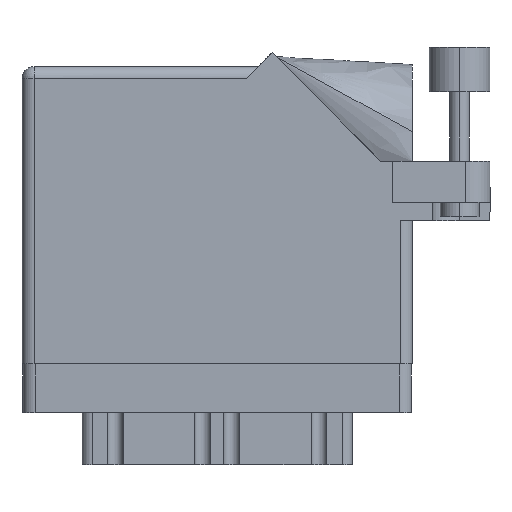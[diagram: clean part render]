
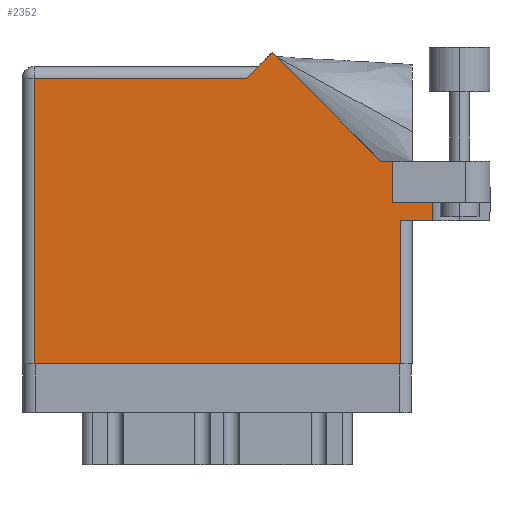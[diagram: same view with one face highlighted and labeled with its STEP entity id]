
A CAD part, front view. The second image highlights one B-rep face of the part: STEP entity #2352.
In plain terms, the highlighted face is planar.
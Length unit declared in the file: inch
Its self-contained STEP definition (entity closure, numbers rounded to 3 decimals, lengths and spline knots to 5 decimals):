
#315 = VERTEX_POINT ( 'NONE', #24231 ) ;
#578 = CARTESIAN_POINT ( 'NONE',  ( 1.155, 1.468, 0. ) ) ;
#921 = VERTEX_POINT ( 'NONE', #22400 ) ;
#976 = LINE ( 'NONE', #22211, #2198 ) ;
#1075 = CARTESIAN_POINT ( 'NONE',  ( 0.062, 0., 0. ) ) ;
#1170 = AXIS2_PLACEMENT_3D ( 'NONE', #5029, #34417, #10353 ) ;
#1180 = VERTEX_POINT ( 'NONE', #21303 ) ;
#1255 = LINE ( 'NONE', #20189, #10059 ) ;
#1613 = EDGE_CURVE ( 'NONE', #1180, #15793, #21962, .T. ) ;
#2024 = LINE ( 'NONE', #17772, #23167 ) ;
#2198 = VECTOR ( 'NONE', #30543, 39.37008 ) ;
#2352 = ADVANCED_FACE ( 'NONE', ( #12845 ), #23617, .F. ) ;
#2527 = DIRECTION ( 'NONE',  ( 0., 1., 0. ) ) ;
#2642 = VECTOR ( 'NONE', #23345, 39.37008 ) ;
#2678 = CARTESIAN_POINT ( 'NONE',  ( 0., 0., 0. ) ) ;
#2795 = CARTESIAN_POINT ( 'NONE',  ( 1.84442, 1.044, 0. ) ) ;
#3023 = CARTESIAN_POINT ( 'NONE',  ( 0.062, 0., 0. ) ) ;
#3387 = EDGE_CURVE ( 'NONE', #32485, #20541, #27053, .T. ) ;
#4125 = LINE ( 'NONE', #12821, #17783 ) ;
#4178 = ORIENTED_EDGE ( 'NONE', *, *, #29573, .T. ) ;
#4871 = ORIENTED_EDGE ( 'NONE', *, *, #3387, .T. ) ;
#5029 = CARTESIAN_POINT ( 'NONE',  ( 0., 1.53, 0. ) ) ;
#5056 = EDGE_CURVE ( 'NONE', #9277, #1180, #976, .T. ) ;
#5704 = CARTESIAN_POINT ( 'NONE',  ( 1.217, 1.53, 0. ) ) ;
#5858 = DIRECTION ( 'NONE',  ( 1., 0., 0. ) ) ;
#6406 = EDGE_CURVE ( 'NONE', #921, #31021, #2024, .T. ) ;
#6915 = CARTESIAN_POINT ( 'NONE',  ( 1.91, 1.044, 0. ) ) ;
#7485 = LINE ( 'NONE', #9984, #20036 ) ;
#8009 = DIRECTION ( 'NONE',  ( -0.707, -0.707, 0. ) ) ;
#8071 = VERTEX_POINT ( 'NONE', #6915 ) ;
#8391 = ORIENTED_EDGE ( 'NONE', *, *, #23736, .F. ) ;
#8511 = VECTOR ( 'NONE', #13611, 39.37008 ) ;
#8590 = DIRECTION ( 'NONE',  ( -1., 0., 0. ) ) ;
#8697 = DIRECTION ( 'NONE',  ( 0., 1., 0. ) ) ;
#9277 = VERTEX_POINT ( 'NONE', #578 ) ;
#9984 = CARTESIAN_POINT ( 'NONE',  ( 1.948, 0.737, 0. ) ) ;
#10059 = VECTOR ( 'NONE', #8697, 39.37008 ) ;
#10234 = CARTESIAN_POINT ( 'NONE',  ( 1.84442, 1.044, 0. ) ) ;
#10353 = DIRECTION ( 'NONE',  ( -1., 0., 0. ) ) ;
#12574 = CARTESIAN_POINT ( 'NONE',  ( 2.01, 0.737, 0. ) ) ;
#12821 = CARTESIAN_POINT ( 'NONE',  ( 2.1115, 1.16177, 0. ) ) ;
#12845 = FACE_OUTER_BOUND ( 'NONE', #19191, .T. ) ;
#13579 = ORIENTED_EDGE ( 'NONE', *, *, #19293, .T. ) ;
#13611 = DIRECTION ( 'NONE',  ( -0.707, 0.707, 0. ) ) ;
#14449 = VECTOR ( 'NONE', #8009, 39.37008 ) ;
#15306 = DIRECTION ( 'NONE',  ( 1., 0., 0. ) ) ;
#15793 = VERTEX_POINT ( 'NONE', #1075 ) ;
#16318 = DIRECTION ( 'NONE',  ( 0., -1., 0. ) ) ;
#16716 = CARTESIAN_POINT ( 'NONE',  ( 1.28771, 1.60071, 0. ) ) ;
#17705 = VECTOR ( 'NONE', #16318, 39.37008 ) ;
#17772 = CARTESIAN_POINT ( 'NONE',  ( 1.91, 0.831, 0. ) ) ;
#17783 = VECTOR ( 'NONE', #22886, 39.37008 ) ;
#18786 = LINE ( 'NONE', #2678, #30575 ) ;
#18927 = VECTOR ( 'NONE', #8590, 39.37008 ) ;
#19001 = LINE ( 'NONE', #5704, #14449 ) ;
#19191 = EDGE_LOOP ( 'NONE', ( #13579, #20153, #23503, #8391, #21828, #19923, #21890, #4871, #4178, #25066, #27024 ) ) ;
#19293 = EDGE_CURVE ( 'NONE', #15793, #315, #18786, .T. ) ;
#19923 = ORIENTED_EDGE ( 'NONE', *, *, #28394, .T. ) ;
#20036 = VECTOR ( 'NONE', #2527, 39.37008 ) ;
#20153 = ORIENTED_EDGE ( 'NONE', *, *, #34497, .T. ) ;
#20189 = CARTESIAN_POINT ( 'NONE',  ( 1.91, 0.831, 0. ) ) ;
#20541 = VERTEX_POINT ( 'NONE', #16716 ) ;
#20775 = VERTEX_POINT ( 'NONE', #30864 ) ;
#21303 = CARTESIAN_POINT ( 'NONE',  ( 0.062, 1.468, 0. ) ) ;
#21828 = ORIENTED_EDGE ( 'NONE', *, *, #6406, .F. ) ;
#21890 = ORIENTED_EDGE ( 'NONE', *, *, #23672, .T. ) ;
#21962 = LINE ( 'NONE', #3023, #17705 ) ;
#22211 = CARTESIAN_POINT ( 'NONE',  ( 0., 1.468, 0. ) ) ;
#22400 = CARTESIAN_POINT ( 'NONE',  ( 1.91, 0.831, 0. ) ) ;
#22886 = DIRECTION ( 'NONE',  ( 0., -1., 0. ) ) ;
#23167 = VECTOR ( 'NONE', #15306, 39.37008 ) ;
#23345 = DIRECTION ( 'NONE',  ( 1., 0., 0. ) ) ;
#23503 = ORIENTED_EDGE ( 'NONE', *, *, #27329, .T. ) ;
#23617 = PLANE ( 'NONE',  #1170 ) ;
#23672 = EDGE_CURVE ( 'NONE', #8071, #32485, #25218, .T. ) ;
#23736 = EDGE_CURVE ( 'NONE', #31021, #20775, #4125, .T. ) ;
#24231 = CARTESIAN_POINT ( 'NONE',  ( 1.948, 0., 0. ) ) ;
#25066 = ORIENTED_EDGE ( 'NONE', *, *, #5056, .T. ) ;
#25218 = LINE ( 'NONE', #32835, #18927 ) ;
#25669 = CARTESIAN_POINT ( 'NONE',  ( 1.948, 0.737, 0. ) ) ;
#26385 = LINE ( 'NONE', #12574, #2642 ) ;
#26763 = CARTESIAN_POINT ( 'NONE',  ( 2.1115, 0.831, 0. ) ) ;
#27024 = ORIENTED_EDGE ( 'NONE', *, *, #1613, .T. ) ;
#27053 = LINE ( 'NONE', #2795, #8511 ) ;
#27329 = EDGE_CURVE ( 'NONE', #31953, #20775, #26385, .T. ) ;
#28394 = EDGE_CURVE ( 'NONE', #921, #8071, #1255, .T. ) ;
#29573 = EDGE_CURVE ( 'NONE', #20541, #9277, #19001, .T. ) ;
#30543 = DIRECTION ( 'NONE',  ( -1., 0., 0. ) ) ;
#30575 = VECTOR ( 'NONE', #5858, 39.37008 ) ;
#30864 = CARTESIAN_POINT ( 'NONE',  ( 2.1115, 0.737, 0. ) ) ;
#31021 = VERTEX_POINT ( 'NONE', #26763 ) ;
#31953 = VERTEX_POINT ( 'NONE', #25669 ) ;
#32485 = VERTEX_POINT ( 'NONE', #10234 ) ;
#32835 = CARTESIAN_POINT ( 'NONE',  ( 2.41, 1.044, 0. ) ) ;
#34417 = DIRECTION ( 'NONE',  ( 0., 0., -1. ) ) ;
#34497 = EDGE_CURVE ( 'NONE', #315, #31953, #7485, .T. ) ;
